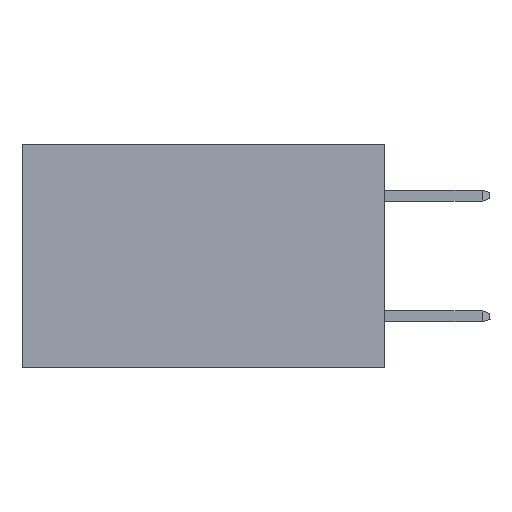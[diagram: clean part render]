
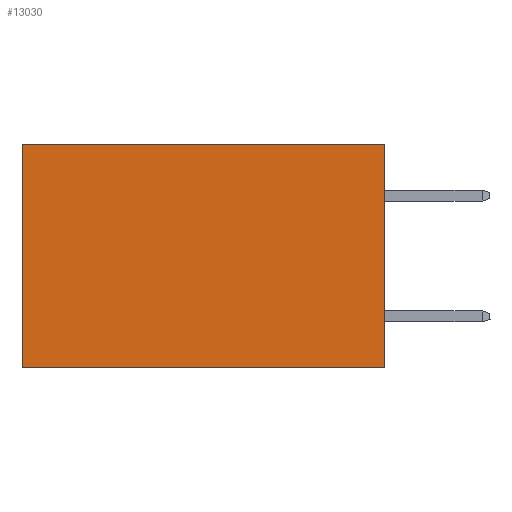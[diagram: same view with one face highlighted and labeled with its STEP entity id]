
A CAD part, left-side view. The second image highlights one B-rep face of the part: STEP entity #13030.
In plain terms, the highlighted planar face has unit normal (-1, 0, 0).
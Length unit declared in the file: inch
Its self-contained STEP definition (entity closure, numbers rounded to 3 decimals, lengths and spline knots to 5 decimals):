
#576 = VECTOR ( 'NONE', #18179, 39.37008 ) ;
#3347 = CARTESIAN_POINT ( 'NONE',  ( 0.2615, 0.6, -0.37 ) ) ;
#4231 = VECTOR ( 'NONE', #10054, 39.37008 ) ;
#5013 = ORIENTED_EDGE ( 'NONE', *, *, #10751, .T. ) ;
#5049 = LINE ( 'NONE', #8808, #17640 ) ;
#5657 = CARTESIAN_POINT ( 'NONE',  ( 0.2615, 0., -0.37 ) ) ;
#5825 = VERTEX_POINT ( 'NONE', #8070 ) ;
#6165 = VERTEX_POINT ( 'NONE', #15557 ) ;
#6506 = CARTESIAN_POINT ( 'NONE',  ( 0.2615, 0., 0. ) ) ;
#6864 = VERTEX_POINT ( 'NONE', #5657 ) ;
#7575 = EDGE_LOOP ( 'NONE', ( #5013, #19813, #15917, #11274 ) ) ;
#8070 = CARTESIAN_POINT ( 'NONE',  ( 0.2615, 0., 0. ) ) ;
#8539 = VECTOR ( 'NONE', #9007, 39.37008 ) ;
#8765 = EDGE_CURVE ( 'NONE', #5825, #6165, #17350, .T. ) ;
#8808 = CARTESIAN_POINT ( 'NONE',  ( 0.2615, 0., -0.37 ) ) ;
#9007 = DIRECTION ( 'NONE',  ( 0., 0., -1. ) ) ;
#9870 = DIRECTION ( 'NONE',  ( 0., 0., -1. ) ) ;
#10054 = DIRECTION ( 'NONE',  ( 0., 0., -1. ) ) ;
#10751 = EDGE_CURVE ( 'NONE', #6165, #13679, #18570, .T. ) ;
#11274 = ORIENTED_EDGE ( 'NONE', *, *, #8765, .T. ) ;
#11358 = CARTESIAN_POINT ( 'NONE',  ( 0.2615, 0.6, -0.37 ) ) ;
#12236 = CARTESIAN_POINT ( 'NONE',  ( 0.2615, 0., -0.37 ) ) ;
#13030 = ADVANCED_FACE ( 'NONE', ( #16337 ), #13135, .F. ) ;
#13135 = PLANE ( 'NONE',  #17700 ) ;
#13679 = VERTEX_POINT ( 'NONE', #11358 ) ;
#15557 = CARTESIAN_POINT ( 'NONE',  ( 0.2615, 0.6, 0. ) ) ;
#15917 = ORIENTED_EDGE ( 'NONE', *, *, #18366, .F. ) ;
#15997 = EDGE_CURVE ( 'NONE', #6864, #13679, #5049, .T. ) ;
#16337 = FACE_OUTER_BOUND ( 'NONE', #7575, .T. ) ;
#16504 = CARTESIAN_POINT ( 'NONE',  ( 0.2615, 0., -0.37 ) ) ;
#17350 = LINE ( 'NONE', #6506, #576 ) ;
#17640 = VECTOR ( 'NONE', #18797, 39.37008 ) ;
#17700 = AXIS2_PLACEMENT_3D ( 'NONE', #16504, #19887, #9870 ) ;
#17964 = LINE ( 'NONE', #12236, #8539 ) ;
#18179 = DIRECTION ( 'NONE',  ( 0., 1., 0. ) ) ;
#18366 = EDGE_CURVE ( 'NONE', #5825, #6864, #17964, .T. ) ;
#18570 = LINE ( 'NONE', #3347, #4231 ) ;
#18797 = DIRECTION ( 'NONE',  ( 0., 1., 0. ) ) ;
#19813 = ORIENTED_EDGE ( 'NONE', *, *, #15997, .F. ) ;
#19887 = DIRECTION ( 'NONE',  ( 1., 0., 0. ) ) ;
